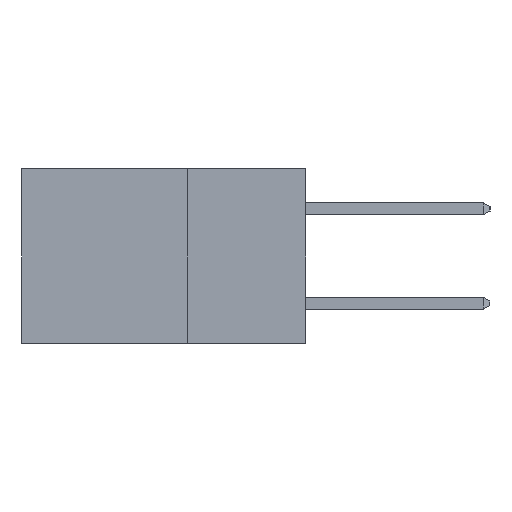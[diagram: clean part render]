
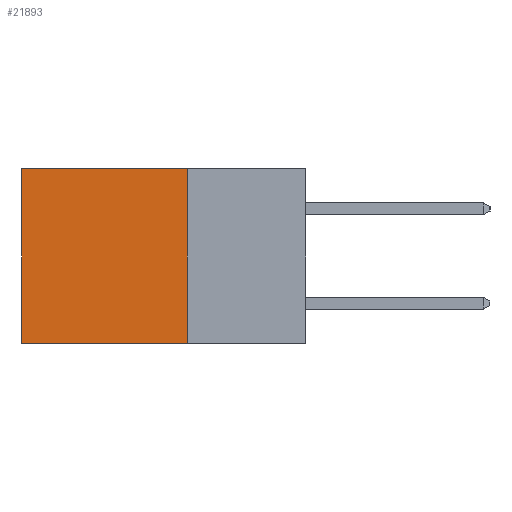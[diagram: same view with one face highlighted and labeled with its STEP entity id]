
A CAD part, left-side view. The second image highlights one B-rep face of the part: STEP entity #21893.
In plain terms, the highlighted planar face has unit normal (-1, 0, 0).
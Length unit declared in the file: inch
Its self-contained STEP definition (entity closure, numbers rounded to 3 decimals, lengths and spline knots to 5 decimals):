
#2225 = DIRECTION ( 'NONE',  ( 0., 1., 0. ) ) ;
#2517 = EDGE_CURVE ( 'NONE', #15646, #2893, #6499, .T. ) ;
#2893 = VERTEX_POINT ( 'NONE', #4632 ) ;
#3514 = VECTOR ( 'NONE', #2225, 39.37008 ) ;
#4141 = LINE ( 'NONE', #6344, #3514 ) ;
#4527 = CARTESIAN_POINT ( 'NONE',  ( 0.2615, 0.25, 0. ) ) ;
#4632 = CARTESIAN_POINT ( 'NONE',  ( 0.2615, 0.25, -0.37 ) ) ;
#4925 = DIRECTION ( 'NONE',  ( 1., 0., 0. ) ) ;
#6084 = CARTESIAN_POINT ( 'NONE',  ( 0.2615, 0.6, 0. ) ) ;
#6344 = CARTESIAN_POINT ( 'NONE',  ( 0.2615, 0.25, -0.37 ) ) ;
#6499 = LINE ( 'NONE', #10722, #6622 ) ;
#6622 = VECTOR ( 'NONE', #8806, 39.37008 ) ;
#6633 = LINE ( 'NONE', #10869, #15018 ) ;
#6778 = ORIENTED_EDGE ( 'NONE', *, *, #22486, .T. ) ;
#7754 = AXIS2_PLACEMENT_3D ( 'NONE', #9043, #4925, #24875 ) ;
#8732 = ORIENTED_EDGE ( 'NONE', *, *, #9544, .F. ) ;
#8806 = DIRECTION ( 'NONE',  ( 0., 0., -1. ) ) ;
#9007 = VECTOR ( 'NONE', #9610, 39.37008 ) ;
#9043 = CARTESIAN_POINT ( 'NONE',  ( 0.2615, 0.25, -0.37 ) ) ;
#9064 = DIRECTION ( 'NONE',  ( 0., 1., 0. ) ) ;
#9544 = EDGE_CURVE ( 'NONE', #2893, #24296, #4141, .T. ) ;
#9610 = DIRECTION ( 'NONE',  ( 0., 0., -1. ) ) ;
#10722 = CARTESIAN_POINT ( 'NONE',  ( 0.2615, 0.25, -0.37 ) ) ;
#10869 = CARTESIAN_POINT ( 'NONE',  ( 0.2615, 0.25, 0. ) ) ;
#13656 = EDGE_CURVE ( 'NONE', #15646, #21664, #6633, .T. ) ;
#14508 = ORIENTED_EDGE ( 'NONE', *, *, #2517, .F. ) ;
#14713 = PLANE ( 'NONE',  #7754 ) ;
#15018 = VECTOR ( 'NONE', #9064, 39.37008 ) ;
#15646 = VERTEX_POINT ( 'NONE', #4527 ) ;
#19233 = CARTESIAN_POINT ( 'NONE',  ( 0.2615, 0.6, -0.37 ) ) ;
#20464 = FACE_OUTER_BOUND ( 'NONE', #24622, .T. ) ;
#21435 = ORIENTED_EDGE ( 'NONE', *, *, #13656, .T. ) ;
#21664 = VERTEX_POINT ( 'NONE', #6084 ) ;
#21893 = ADVANCED_FACE ( 'NONE', ( #20464 ), #14713, .F. ) ;
#22486 = EDGE_CURVE ( 'NONE', #21664, #24296, #25302, .T. ) ;
#23508 = CARTESIAN_POINT ( 'NONE',  ( 0.2615, 0.6, -0.37 ) ) ;
#24296 = VERTEX_POINT ( 'NONE', #19233 ) ;
#24622 = EDGE_LOOP ( 'NONE', ( #6778, #8732, #14508, #21435 ) ) ;
#24875 = DIRECTION ( 'NONE',  ( 0., 0., -1. ) ) ;
#25302 = LINE ( 'NONE', #23508, #9007 ) ;
